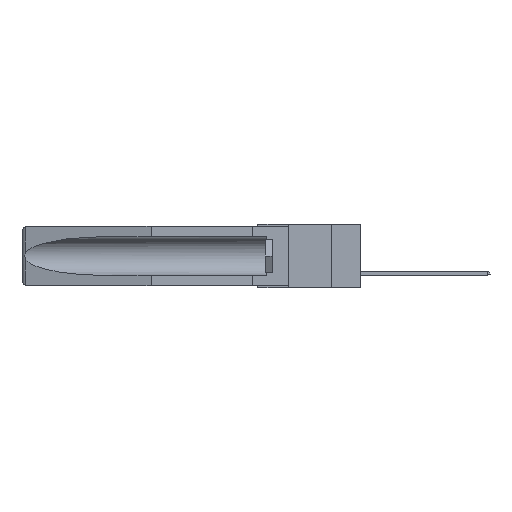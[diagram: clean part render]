
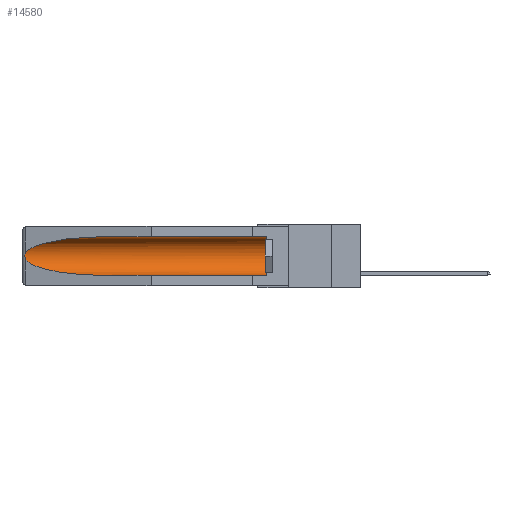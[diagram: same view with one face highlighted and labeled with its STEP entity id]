
A CAD part, left-side view. The second image highlights one B-rep face of the part: STEP entity #14580.
In plain terms, the highlighted cylindrical face has radius 2.857 mm (diameter 5.715 mm), a partial arc.
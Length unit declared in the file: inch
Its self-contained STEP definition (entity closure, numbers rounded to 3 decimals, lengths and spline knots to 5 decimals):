
#87 = VECTOR ( 'NONE', #23209, 39.37008 ) ;
#675 = EDGE_LOOP ( 'NONE', ( #1148, #785, #10928, #20265, #11176, #1052 ) ) ;
#785 = ORIENTED_EDGE ( 'NONE', *, *, #3033, .T. ) ;
#1052 = ORIENTED_EDGE ( 'NONE', *, *, #13709, .T. ) ;
#1148 = ORIENTED_EDGE ( 'NONE', *, *, #12955, .T. ) ;
#1222 = CARTESIAN_POINT ( 'NONE',  ( 0.155, 0.126, -0.1715 ) ) ;
#1861 = CARTESIAN_POINT ( 'NONE',  ( 0.26537, 1.52718, -0.14972 ) ) ;
#1879 = CARTESIAN_POINT ( 'NONE',  ( 0.155, 1.07973, -0.284 ) ) ;
#2261 = CARTESIAN_POINT ( 'NONE',  ( 0.2673, 1.5327, -0.16383 ) ) ;
#2484 = AXIS2_PLACEMENT_3D ( 'NONE', #18150, #2909, #4156 ) ;
#2909 = DIRECTION ( 'NONE',  ( 0., 1., 0. ) ) ;
#3033 = EDGE_CURVE ( 'NONE', #25861, #3653, #19080, .T. ) ;
#3273 = CARTESIAN_POINT ( 'NONE',  ( 0.155, 0.126, -0.284 ) ) ;
#3653 = VERTEX_POINT ( 'NONE', #29510 ) ;
#4156 = DIRECTION ( 'NONE',  ( 0., 0., 1. ) ) ;
#4546 = CARTESIAN_POINT ( 'NONE',  ( 0.26537, 1.52718, -0.19328 ) ) ;
#5369 = EDGE_CURVE ( 'NONE', #3653, #9266, #26228, .T. ) ;
#6180 = VECTOR ( 'NONE', #22710, 39.37008 ) ;
#6195 = CARTESIAN_POINT ( 'NONE',  ( 0.26537, 1.52718, -0.14972 ) ) ;
#6310 = CARTESIAN_POINT ( 'NONE',  ( 0.25451, 1.48313, -0.09465 ) ) ;
#6625 = CARTESIAN_POINT ( 'NONE',  ( 0.26655, 1.53094, -0.18657 ) ) ;
#7076 = CARTESIAN_POINT ( 'NONE',  ( 0.155, -0.30754, -0.284 ) ) ;
#7740 =( BOUNDED_CURVE ( )  B_SPLINE_CURVE ( 3, ( #15406, #8405, #6310, #22456 ),
 .UNSPECIFIED., .F., .F. ) 
 B_SPLINE_CURVE_WITH_KNOTS ( ( 4, 4 ),
 ( 4.71239, 6.08839 ),
 .UNSPECIFIED. ) 
 CURVE ( )  GEOMETRIC_REPRESENTATION_ITEM ( )  RATIONAL_B_SPLINE_CURVE ( ( 1., 0.848, 0.848, 1. ) ) 
 REPRESENTATION_ITEM ( '' )  );
#7799 = EDGE_CURVE ( 'NONE', #24346, #9266, #18982, .T. ) ;
#8212 = CARTESIAN_POINT ( 'NONE',  ( 0.155, 0.126, -0.059 ) ) ;
#8405 = CARTESIAN_POINT ( 'NONE',  ( 0.21114, 1.30732, -0.059 ) ) ;
#9210 = EDGE_CURVE ( 'NONE', #24346, #10983, #11097, .T. ) ;
#9266 = VERTEX_POINT ( 'NONE', #1879 ) ;
#10928 = ORIENTED_EDGE ( 'NONE', *, *, #5369, .T. ) ;
#10983 = VERTEX_POINT ( 'NONE', #8212 ) ;
#11097 = CIRCLE ( 'NONE', #19204, 0.1125 ) ;
#11122 = CARTESIAN_POINT ( 'NONE',  ( 0.2675, 1.53308, -0.16763 ) ) ;
#11167 = CARTESIAN_POINT ( 'NONE',  ( 0.26537, 1.52718, -0.19328 ) ) ;
#11176 = ORIENTED_EDGE ( 'NONE', *, *, #9210, .T. ) ;
#12679 = DIRECTION ( 'NONE',  ( 0., -1., 0. ) ) ;
#12955 = EDGE_CURVE ( 'NONE', #12994, #25861, #7740, .T. ) ;
#12994 = VERTEX_POINT ( 'NONE', #13214 ) ;
#13214 = CARTESIAN_POINT ( 'NONE',  ( 0.155, 1.07973, -0.059 ) ) ;
#13545 = CARTESIAN_POINT ( 'NONE',  ( 0.155, -0.30754, -0.059 ) ) ;
#13709 = EDGE_CURVE ( 'NONE', #10983, #12994, #28304, .T. ) ;
#14580 = ADVANCED_FACE ( 'NONE', ( #20407 ), #23263, .F. ) ;
#15406 = CARTESIAN_POINT ( 'NONE',  ( 0.155, 1.07973, -0.059 ) ) ;
#15526 = CARTESIAN_POINT ( 'NONE',  ( 0.2673, 1.53269, -0.17917 ) ) ;
#15667 = CARTESIAN_POINT ( 'NONE',  ( 0.25451, 1.48313, -0.24835 ) ) ;
#18021 = CARTESIAN_POINT ( 'NONE',  ( 0.26597, 1.52961, -0.15275 ) ) ;
#18109 = CARTESIAN_POINT ( 'NONE',  ( 0.26654, 1.53092, -0.15636 ) ) ;
#18150 = CARTESIAN_POINT ( 'NONE',  ( 0.155, -0.30754, -0.1715 ) ) ;
#18982 = LINE ( 'NONE', #7076, #87 ) ;
#19080 = B_SPLINE_CURVE_WITH_KNOTS ( 'NONE', 3,
 ( #1861, #18021, #18109, #2261, #11122, #29139, #15526, #6625, #20082, #4546 ),
 .UNSPECIFIED., .F., .F.,
 ( 4, 2, 2, 2, 4 ),
 ( 0., 0.00029, 0.00058, 0.00087, 0.00117 ),
 .UNSPECIFIED. ) ;
#19204 = AXIS2_PLACEMENT_3D ( 'NONE', #1222, #12679, #28601 ) ;
#20082 = CARTESIAN_POINT ( 'NONE',  ( 0.26597, 1.5296, -0.19026 ) ) ;
#20265 = ORIENTED_EDGE ( 'NONE', *, *, #7799, .F. ) ;
#20407 = FACE_OUTER_BOUND ( 'NONE', #675, .T. ) ;
#20439 = CARTESIAN_POINT ( 'NONE',  ( 0.155, 1.07973, -0.284 ) ) ;
#22456 = CARTESIAN_POINT ( 'NONE',  ( 0.26537, 1.52718, -0.14972 ) ) ;
#22710 = DIRECTION ( 'NONE',  ( 0., 1., 0. ) ) ;
#23209 = DIRECTION ( 'NONE',  ( 0., 1., 0. ) ) ;
#23263 = CYLINDRICAL_SURFACE ( 'NONE', #2484, 0.1125 ) ;
#24346 = VERTEX_POINT ( 'NONE', #3273 ) ;
#25861 = VERTEX_POINT ( 'NONE', #6195 ) ;
#26228 =( BOUNDED_CURVE ( )  B_SPLINE_CURVE ( 3, ( #11167, #15667, #27298, #20439 ),
 .UNSPECIFIED., .F., .F. ) 
 B_SPLINE_CURVE_WITH_KNOTS ( ( 4, 4 ),
 ( 0.1948, 1.5708 ),
 .UNSPECIFIED. ) 
 CURVE ( )  GEOMETRIC_REPRESENTATION_ITEM ( )  RATIONAL_B_SPLINE_CURVE ( ( 1., 0.848, 0.848, 1. ) ) 
 REPRESENTATION_ITEM ( '' )  );
#27298 = CARTESIAN_POINT ( 'NONE',  ( 0.21114, 1.30732, -0.284 ) ) ;
#28304 = LINE ( 'NONE', #13545, #6180 ) ;
#28601 = DIRECTION ( 'NONE',  ( 0., 0., 1. ) ) ;
#29139 = CARTESIAN_POINT ( 'NONE',  ( 0.2675, 1.53308, -0.17534 ) ) ;
#29510 = CARTESIAN_POINT ( 'NONE',  ( 0.26537, 1.52718, -0.19328 ) ) ;
